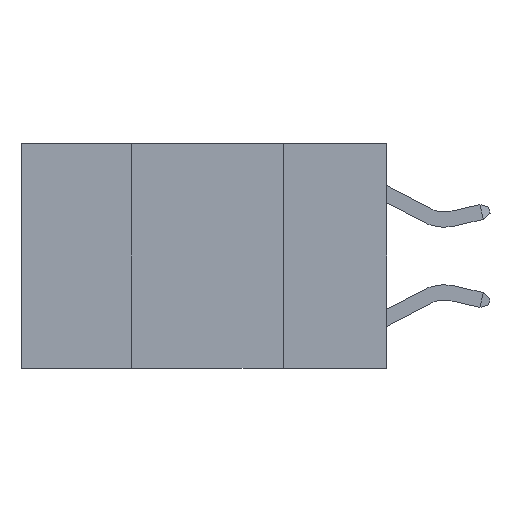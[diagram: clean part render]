
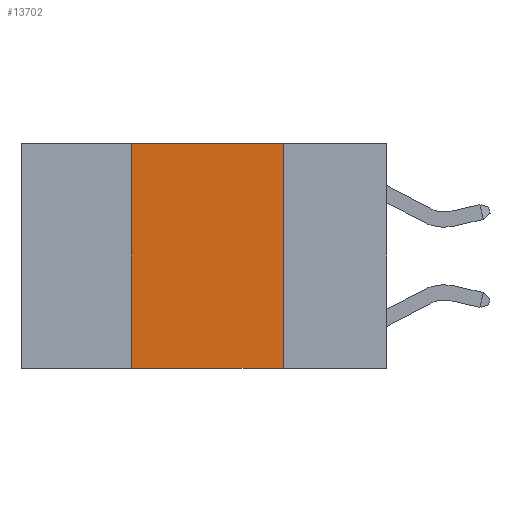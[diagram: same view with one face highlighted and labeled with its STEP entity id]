
A CAD part, left-side view. The second image highlights one B-rep face of the part: STEP entity #13702.
In plain terms, the highlighted planar face has unit normal (-1, 0, 0).
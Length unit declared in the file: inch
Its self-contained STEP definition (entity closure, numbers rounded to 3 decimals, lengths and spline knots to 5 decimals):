
#738 = CARTESIAN_POINT ( 'NONE',  ( 0., 0.17, 0. ) ) ;
#1575 = ORIENTED_EDGE ( 'NONE', *, *, #10748, .T. ) ;
#2538 = EDGE_CURVE ( 'NONE', #2700, #4733, #18397, .T. ) ;
#2543 = VECTOR ( 'NONE', #6903, 39.37008 ) ;
#2700 = VERTEX_POINT ( 'NONE', #11158 ) ;
#3038 = CARTESIAN_POINT ( 'NONE',  ( 0., 0.6, 0. ) ) ;
#3215 = AXIS2_PLACEMENT_3D ( 'NONE', #8700, #19402, #10226 ) ;
#3805 = LINE ( 'NONE', #15623, #7505 ) ;
#3930 = LINE ( 'NONE', #3038, #15857 ) ;
#3949 = PLANE ( 'NONE',  #3215 ) ;
#4639 = DIRECTION ( 'NONE',  ( 0., -1., 0. ) ) ;
#4733 = VERTEX_POINT ( 'NONE', #6249 ) ;
#6249 = CARTESIAN_POINT ( 'NONE',  ( 0., 0.42, 0. ) ) ;
#6753 = LINE ( 'NONE', #738, #2543 ) ;
#6903 = DIRECTION ( 'NONE',  ( 0., 0., -1. ) ) ;
#7404 = VERTEX_POINT ( 'NONE', #16452 ) ;
#7505 = VECTOR ( 'NONE', #7922, 39.37008 ) ;
#7922 = DIRECTION ( 'NONE',  ( 0., -1., 0. ) ) ;
#8474 = ORIENTED_EDGE ( 'NONE', *, *, #17389, .F. ) ;
#8700 = CARTESIAN_POINT ( 'NONE',  ( 0., 0.6, 0. ) ) ;
#8858 = FACE_OUTER_BOUND ( 'NONE', #17928, .T. ) ;
#8940 = ORIENTED_EDGE ( 'NONE', *, *, #14007, .F. ) ;
#9018 = VERTEX_POINT ( 'NONE', #14449 ) ;
#9260 = DIRECTION ( 'NONE',  ( 0., 0., 1. ) ) ;
#10226 = DIRECTION ( 'NONE',  ( 0., 0., -1. ) ) ;
#10701 = VECTOR ( 'NONE', #9260, 39.37008 ) ;
#10748 = EDGE_CURVE ( 'NONE', #2700, #9018, #3805, .T. ) ;
#11158 = CARTESIAN_POINT ( 'NONE',  ( 0., 0.42, -0.37 ) ) ;
#13702 = ADVANCED_FACE ( 'NONE', ( #8858 ), #3949, .F. ) ;
#14007 = EDGE_CURVE ( 'NONE', #4733, #7404, #3930, .T. ) ;
#14449 = CARTESIAN_POINT ( 'NONE',  ( 0., 0.17, -0.37 ) ) ;
#15623 = CARTESIAN_POINT ( 'NONE',  ( 0., 0.6, -0.37 ) ) ;
#15857 = VECTOR ( 'NONE', #4639, 39.37008 ) ;
#16452 = CARTESIAN_POINT ( 'NONE',  ( 0., 0.17, 0. ) ) ;
#17389 = EDGE_CURVE ( 'NONE', #7404, #9018, #6753, .T. ) ;
#17611 = ORIENTED_EDGE ( 'NONE', *, *, #2538, .F. ) ;
#17928 = EDGE_LOOP ( 'NONE', ( #8474, #8940, #17611, #1575 ) ) ;
#18397 = LINE ( 'NONE', #19956, #10701 ) ;
#19402 = DIRECTION ( 'NONE',  ( 1., 0., 0. ) ) ;
#19956 = CARTESIAN_POINT ( 'NONE',  ( 0., 0.42, 0. ) ) ;
